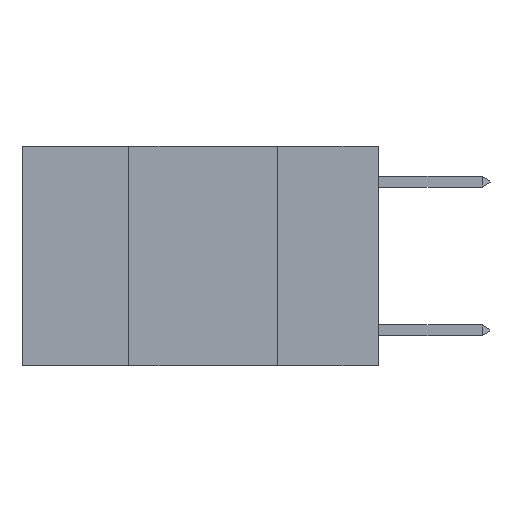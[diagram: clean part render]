
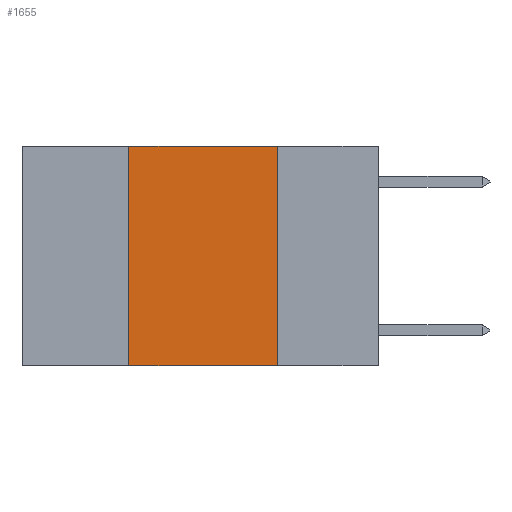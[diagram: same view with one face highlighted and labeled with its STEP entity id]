
A CAD part, left-side view. The second image highlights one B-rep face of the part: STEP entity #1655.
In plain terms, the highlighted planar face has unit normal (-1, 0, 0).
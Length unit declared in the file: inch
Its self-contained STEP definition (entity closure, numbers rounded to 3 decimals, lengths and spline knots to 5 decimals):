
#90 = CARTESIAN_POINT ( 'NONE',  ( 0., 0.42, 0. ) ) ;
#824 = VERTEX_POINT ( 'NONE', #13084 ) ;
#1384 = EDGE_CURVE ( 'NONE', #7412, #20933, #4156, .T. ) ;
#1655 = ADVANCED_FACE ( 'NONE', ( #3874 ), #1836, .F. ) ;
#1759 = DIRECTION ( 'NONE',  ( 0., 0., -1. ) ) ;
#1782 = DIRECTION ( 'NONE',  ( 1., 0., 0. ) ) ;
#1836 = PLANE ( 'NONE',  #20907 ) ;
#2121 = CARTESIAN_POINT ( 'NONE',  ( 0., 0.6, 0. ) ) ;
#2166 = CARTESIAN_POINT ( 'NONE',  ( 0., 0.42, -0.37 ) ) ;
#3105 = CARTESIAN_POINT ( 'NONE',  ( 0., 0.17, -0.37 ) ) ;
#3874 = FACE_OUTER_BOUND ( 'NONE', #11482, .T. ) ;
#4156 = LINE ( 'NONE', #5374, #9424 ) ;
#4182 = ORIENTED_EDGE ( 'NONE', *, *, #4992, .F. ) ;
#4625 = VECTOR ( 'NONE', #10664, 39.37008 ) ;
#4965 = EDGE_CURVE ( 'NONE', #7613, #824, #16328, .T. ) ;
#4992 = EDGE_CURVE ( 'NONE', #7412, #7613, #11105, .T. ) ;
#5374 = CARTESIAN_POINT ( 'NONE',  ( 0., 0.6, -0.37 ) ) ;
#5431 = DIRECTION ( 'NONE',  ( 0., -1., 0. ) ) ;
#6461 = VECTOR ( 'NONE', #10580, 39.37008 ) ;
#7412 = VERTEX_POINT ( 'NONE', #2166 ) ;
#7613 = VERTEX_POINT ( 'NONE', #90 ) ;
#8579 = EDGE_CURVE ( 'NONE', #824, #20933, #14002, .T. ) ;
#9424 = VECTOR ( 'NONE', #5431, 39.37008 ) ;
#10298 = CARTESIAN_POINT ( 'NONE',  ( 0., 0.17, 0. ) ) ;
#10580 = DIRECTION ( 'NONE',  ( 0., 0., 1. ) ) ;
#10664 = DIRECTION ( 'NONE',  ( 0., 0., -1. ) ) ;
#10902 = CARTESIAN_POINT ( 'NONE',  ( 0., 0.42, 0. ) ) ;
#10972 = ORIENTED_EDGE ( 'NONE', *, *, #8579, .F. ) ;
#11105 = LINE ( 'NONE', #10902, #6461 ) ;
#11145 = DIRECTION ( 'NONE',  ( 0., -1., 0. ) ) ;
#11482 = EDGE_LOOP ( 'NONE', ( #10972, #16460, #4182, #14387 ) ) ;
#11640 = CARTESIAN_POINT ( 'NONE',  ( 0., 0.6, 0. ) ) ;
#13084 = CARTESIAN_POINT ( 'NONE',  ( 0., 0.17, 0. ) ) ;
#14002 = LINE ( 'NONE', #10298, #4625 ) ;
#14387 = ORIENTED_EDGE ( 'NONE', *, *, #1384, .T. ) ;
#16328 = LINE ( 'NONE', #11640, #20341 ) ;
#16460 = ORIENTED_EDGE ( 'NONE', *, *, #4965, .F. ) ;
#20341 = VECTOR ( 'NONE', #11145, 39.37008 ) ;
#20907 = AXIS2_PLACEMENT_3D ( 'NONE', #2121, #1782, #1759 ) ;
#20933 = VERTEX_POINT ( 'NONE', #3105 ) ;
